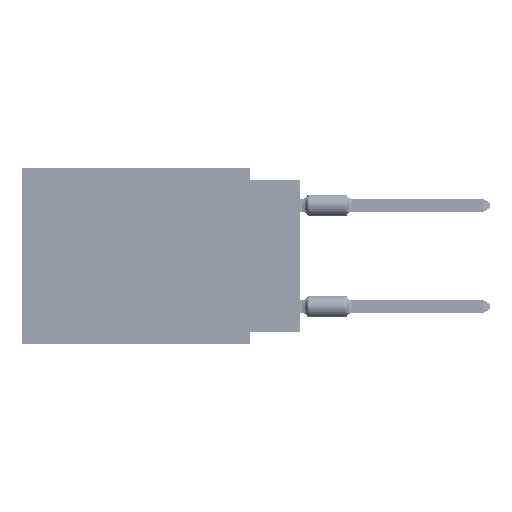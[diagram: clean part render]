
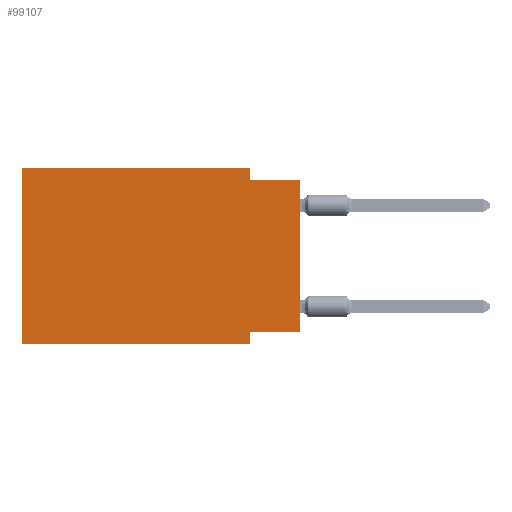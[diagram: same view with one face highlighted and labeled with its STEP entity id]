
A CAD part, left-side view. The second image highlights one B-rep face of the part: STEP entity #99107.
In plain terms, the highlighted planar face has unit normal (-1, 0, 0).
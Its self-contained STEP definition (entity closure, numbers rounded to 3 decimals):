
#351 = DIRECTION ( 'NONE',  ( 1., 0., 0. ) ) ;
#1220 = ORIENTED_EDGE ( 'NONE', *, *, #51631, .F. ) ;
#3698 = CARTESIAN_POINT ( 'NONE',  ( 0., 2.54, -8.255 ) ) ;
#5139 = CARTESIAN_POINT ( 'NONE',  ( 0., 0., 0. ) ) ;
#5437 = VERTEX_POINT ( 'NONE', #95035 ) ;
#6488 = EDGE_CURVE ( 'NONE', #97160, #5437, #105796, .T. ) ;
#8886 = DIRECTION ( 'NONE',  ( 0., 0., 1. ) ) ;
#12979 = LINE ( 'NONE', #71602, #44736 ) ;
#13865 = VECTOR ( 'NONE', #21332, 1000. ) ;
#14603 = LINE ( 'NONE', #62740, #75227 ) ;
#15265 = AXIS2_PLACEMENT_3D ( 'NONE', #34632, #351, #50121 ) ;
#16415 = FACE_OUTER_BOUND ( 'NONE', #28016, .T. ) ;
#18262 = CARTESIAN_POINT ( 'NONE',  ( 0., 13.97, 0. ) ) ;
#21332 = DIRECTION ( 'NONE',  ( 0., -1., 0. ) ) ;
#21871 = CARTESIAN_POINT ( 'NONE',  ( 0., 13.97, 0. ) ) ;
#23809 = VECTOR ( 'NONE', #55600, 1000. ) ;
#28016 = EDGE_LOOP ( 'NONE', ( #48634, #104366, #64735, #64685, #1220, #46286, #58041, #61570 ) ) ;
#30037 = CARTESIAN_POINT ( 'NONE',  ( 0., 0., -8.255 ) ) ;
#30639 = DIRECTION ( 'NONE',  ( 0., 0., -1. ) ) ;
#31002 = CARTESIAN_POINT ( 'NONE',  ( 0., 2.54, 0. ) ) ;
#34632 = CARTESIAN_POINT ( 'NONE',  ( 0., 13.97, 0. ) ) ;
#35035 = EDGE_CURVE ( 'NONE', #69264, #85780, #105950, .T. ) ;
#36150 = VECTOR ( 'NONE', #38858, 1000. ) ;
#36270 = LINE ( 'NONE', #47305, #13865 ) ;
#38814 = LINE ( 'NONE', #70926, #90931 ) ;
#38858 = DIRECTION ( 'NONE',  ( 0., 0., 1. ) ) ;
#41834 = PLANE ( 'NONE',  #15265 ) ;
#44736 = VECTOR ( 'NONE', #30639, 1000. ) ;
#46286 = ORIENTED_EDGE ( 'NONE', *, *, #64868, .T. ) ;
#47163 = VERTEX_POINT ( 'NONE', #81969 ) ;
#47305 = CARTESIAN_POINT ( 'NONE',  ( 0., 13.97, -8.89 ) ) ;
#48634 = ORIENTED_EDGE ( 'NONE', *, *, #6488, .T. ) ;
#49371 = EDGE_CURVE ( 'NONE', #72869, #55598, #12979, .T. ) ;
#50121 = DIRECTION ( 'NONE',  ( 0., 0., -1. ) ) ;
#51631 = EDGE_CURVE ( 'NONE', #47163, #69264, #96612, .T. ) ;
#52219 = EDGE_CURVE ( 'NONE', #55152, #5437, #14603, .T. ) ;
#55026 = CARTESIAN_POINT ( 'NONE',  ( 0., 2.54, -0.635 ) ) ;
#55152 = VERTEX_POINT ( 'NONE', #55026 ) ;
#55598 = VERTEX_POINT ( 'NONE', #83275 ) ;
#55600 = DIRECTION ( 'NONE',  ( 0., -1., 0. ) ) ;
#57348 = VECTOR ( 'NONE', #79179, 1000. ) ;
#58041 = ORIENTED_EDGE ( 'NONE', *, *, #49371, .F. ) ;
#61570 = ORIENTED_EDGE ( 'NONE', *, *, #78677, .F. ) ;
#62740 = CARTESIAN_POINT ( 'NONE',  ( 0., 0., -0.635 ) ) ;
#63292 = DIRECTION ( 'NONE',  ( 0., -1., 0. ) ) ;
#64685 = ORIENTED_EDGE ( 'NONE', *, *, #35035, .F. ) ;
#64735 = ORIENTED_EDGE ( 'NONE', *, *, #79739, .F. ) ;
#64868 = EDGE_CURVE ( 'NONE', #47163, #55598, #36270, .T. ) ;
#69264 = VERTEX_POINT ( 'NONE', #18262 ) ;
#70622 = CARTESIAN_POINT ( 'NONE',  ( 0., 13.97, 0. ) ) ;
#70926 = CARTESIAN_POINT ( 'NONE',  ( 0., 0., -8.255 ) ) ;
#71602 = CARTESIAN_POINT ( 'NONE',  ( 0., 2.54, -8.89 ) ) ;
#71951 = LINE ( 'NONE', #31002, #57348 ) ;
#72869 = VERTEX_POINT ( 'NONE', #3698 ) ;
#75227 = VECTOR ( 'NONE', #63292, 1000. ) ;
#78677 = EDGE_CURVE ( 'NONE', #97160, #72869, #38814, .T. ) ;
#79179 = DIRECTION ( 'NONE',  ( 0., 0., -1. ) ) ;
#79739 = EDGE_CURVE ( 'NONE', #85780, #55152, #71951, .T. ) ;
#81969 = CARTESIAN_POINT ( 'NONE',  ( 0., 13.97, -8.89 ) ) ;
#83275 = CARTESIAN_POINT ( 'NONE',  ( 0., 2.54, -8.89 ) ) ;
#85780 = VERTEX_POINT ( 'NONE', #93097 ) ;
#89286 = VECTOR ( 'NONE', #8886, 1000. ) ;
#90931 = VECTOR ( 'NONE', #104127, 1000. ) ;
#93097 = CARTESIAN_POINT ( 'NONE',  ( 0., 2.54, 0. ) ) ;
#95035 = CARTESIAN_POINT ( 'NONE',  ( 0., 0., -0.635 ) ) ;
#96612 = LINE ( 'NONE', #70622, #89286 ) ;
#97160 = VERTEX_POINT ( 'NONE', #30037 ) ;
#99107 = ADVANCED_FACE ( 'NONE', ( #16415 ), #41834, .F. ) ;
#104127 = DIRECTION ( 'NONE',  ( 0., 1., 0. ) ) ;
#104366 = ORIENTED_EDGE ( 'NONE', *, *, #52219, .F. ) ;
#105796 = LINE ( 'NONE', #5139, #36150 ) ;
#105950 = LINE ( 'NONE', #21871, #23809 ) ;
